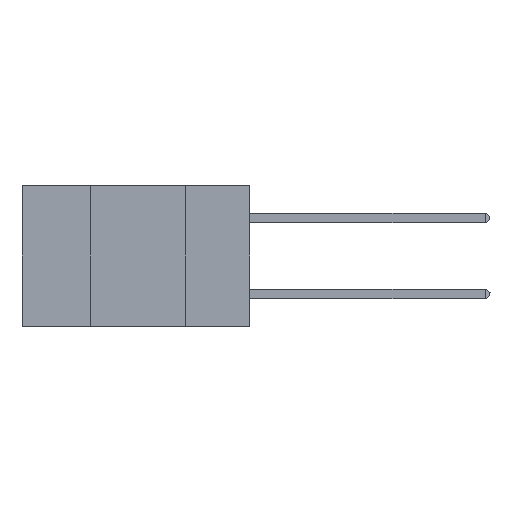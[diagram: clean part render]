
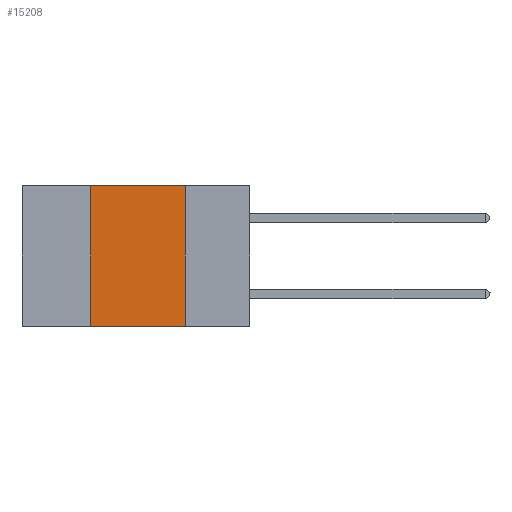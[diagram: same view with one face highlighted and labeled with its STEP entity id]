
A CAD part, left-side view. The second image highlights one B-rep face of the part: STEP entity #15208.
In plain terms, the highlighted planar face has unit normal (-1, 0, 0).
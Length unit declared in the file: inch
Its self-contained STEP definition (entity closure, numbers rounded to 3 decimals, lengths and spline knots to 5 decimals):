
#371 = CARTESIAN_POINT ( 'NONE',  ( 0., 0.17, 0. ) ) ;
#3302 = LINE ( 'NONE', #9468, #16450 ) ;
#4770 = ORIENTED_EDGE ( 'NONE', *, *, #26405, .F. ) ;
#4771 = CARTESIAN_POINT ( 'NONE',  ( 0., 0.6, 0. ) ) ;
#5069 = EDGE_LOOP ( 'NONE', ( #5741, #9512, #4770, #22910 ) ) ;
#5741 = ORIENTED_EDGE ( 'NONE', *, *, #14807, .F. ) ;
#6383 = EDGE_CURVE ( 'NONE', #7447, #12631, #11197, .T. ) ;
#6613 = CARTESIAN_POINT ( 'NONE',  ( 0., 0.6, -0.37 ) ) ;
#7221 = LINE ( 'NONE', #371, #24160 ) ;
#7447 = VERTEX_POINT ( 'NONE', #11040 ) ;
#8558 = PLANE ( 'NONE',  #25733 ) ;
#9468 = CARTESIAN_POINT ( 'NONE',  ( 0., 0.42, 0. ) ) ;
#9512 = ORIENTED_EDGE ( 'NONE', *, *, #20951, .F. ) ;
#9815 = DIRECTION ( 'NONE',  ( 0., 0., 1. ) ) ;
#10043 = CARTESIAN_POINT ( 'NONE',  ( 0., 0.17, 0. ) ) ;
#10311 = CARTESIAN_POINT ( 'NONE',  ( 0., 0.17, -0.37 ) ) ;
#10409 = DIRECTION ( 'NONE',  ( 0., 0., -1. ) ) ;
#10535 = DIRECTION ( 'NONE',  ( 0., -1., 0. ) ) ;
#10991 = DIRECTION ( 'NONE',  ( 0., 0., -1. ) ) ;
#11040 = CARTESIAN_POINT ( 'NONE',  ( 0., 0.42, -0.37 ) ) ;
#11197 = LINE ( 'NONE', #6613, #17585 ) ;
#11434 = VERTEX_POINT ( 'NONE', #15025 ) ;
#12631 = VERTEX_POINT ( 'NONE', #10311 ) ;
#13278 = FACE_OUTER_BOUND ( 'NONE', #5069, .T. ) ;
#14807 = EDGE_CURVE ( 'NONE', #20379, #12631, #7221, .T. ) ;
#15025 = CARTESIAN_POINT ( 'NONE',  ( 0., 0.42, 0. ) ) ;
#15208 = ADVANCED_FACE ( 'NONE', ( #13278 ), #8558, .F. ) ;
#16450 = VECTOR ( 'NONE', #9815, 39.37008 ) ;
#17457 = LINE ( 'NONE', #24974, #20330 ) ;
#17585 = VECTOR ( 'NONE', #24943, 39.37008 ) ;
#20330 = VECTOR ( 'NONE', #10535, 39.37008 ) ;
#20379 = VERTEX_POINT ( 'NONE', #10043 ) ;
#20951 = EDGE_CURVE ( 'NONE', #11434, #20379, #17457, .T. ) ;
#21172 = DIRECTION ( 'NONE',  ( 1., 0., 0. ) ) ;
#22910 = ORIENTED_EDGE ( 'NONE', *, *, #6383, .T. ) ;
#24160 = VECTOR ( 'NONE', #10409, 39.37008 ) ;
#24943 = DIRECTION ( 'NONE',  ( 0., -1., 0. ) ) ;
#24974 = CARTESIAN_POINT ( 'NONE',  ( 0., 0.6, 0. ) ) ;
#25733 = AXIS2_PLACEMENT_3D ( 'NONE', #4771, #21172, #10991 ) ;
#26405 = EDGE_CURVE ( 'NONE', #7447, #11434, #3302, .T. ) ;
